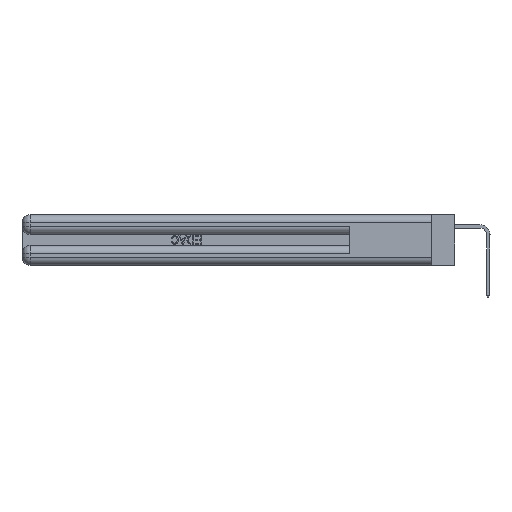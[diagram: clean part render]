
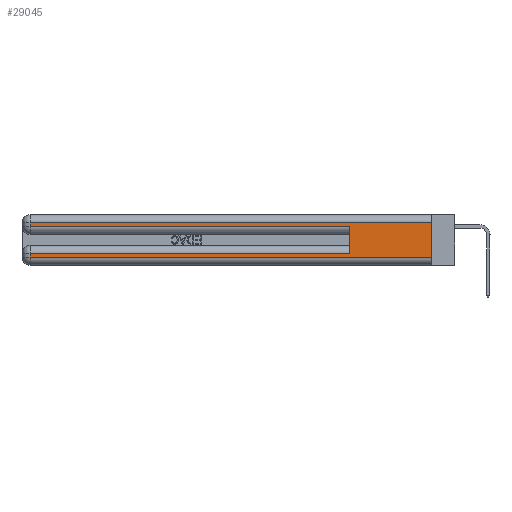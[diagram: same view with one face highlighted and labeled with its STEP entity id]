
A CAD part, left-side view. The second image highlights one B-rep face of the part: STEP entity #29045.
In plain terms, the highlighted planar face has unit normal (-1, 0, 0).
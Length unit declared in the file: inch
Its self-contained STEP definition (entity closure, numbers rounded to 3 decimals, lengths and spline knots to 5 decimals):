
#1526 = ORIENTED_EDGE ( 'NONE', *, *, #7261, .T. ) ;
#1816 = VECTOR ( 'NONE', #19132, 39.37008 ) ;
#1903 = CARTESIAN_POINT ( 'NONE',  ( 0., 0., 0.37 ) ) ;
#2452 = AXIS2_PLACEMENT_3D ( 'NONE', #1903, #26279, #5485 ) ;
#2534 = LINE ( 'NONE', #17965, #29195 ) ;
#3054 = CARTESIAN_POINT ( 'NONE',  ( 0., 0., 0.285 ) ) ;
#3114 = CARTESIAN_POINT ( 'NONE',  ( 0., 2.94, 0.31 ) ) ;
#4350 = ORIENTED_EDGE ( 'NONE', *, *, #4807, .T. ) ;
#4807 = EDGE_CURVE ( 'NONE', #5968, #43733, #16655, .T. ) ;
#5485 = DIRECTION ( 'NONE',  ( 0., 0., -1. ) ) ;
#5968 = VERTEX_POINT ( 'NONE', #27618 ) ;
#6203 = VECTOR ( 'NONE', #27999, 39.37008 ) ;
#6628 = VERTEX_POINT ( 'NONE', #16978 ) ;
#7261 = EDGE_CURVE ( 'NONE', #43733, #33005, #9951, .T. ) ;
#7326 = LINE ( 'NONE', #21052, #6203 ) ;
#8988 = ORIENTED_EDGE ( 'NONE', *, *, #22505, .T. ) ;
#9951 = LINE ( 'NONE', #16258, #11030 ) ;
#10003 = CARTESIAN_POINT ( 'NONE',  ( 0., 0., 0.085 ) ) ;
#10111 = CARTESIAN_POINT ( 'NONE',  ( 0., 2.94, 0.06 ) ) ;
#11030 = VECTOR ( 'NONE', #37002, 39.37008 ) ;
#12995 = EDGE_CURVE ( 'NONE', #5968, #6628, #2534, .T. ) ;
#13821 = CARTESIAN_POINT ( 'NONE',  ( 0., 2.94, 0.285 ) ) ;
#15645 = CARTESIAN_POINT ( 'NONE',  ( 0., 0., 0.06 ) ) ;
#16163 = VERTEX_POINT ( 'NONE', #34158 ) ;
#16258 = CARTESIAN_POINT ( 'NONE',  ( 0., 2.94, 0.37 ) ) ;
#16274 = ORIENTED_EDGE ( 'NONE', *, *, #19928, .T. ) ;
#16655 = LINE ( 'NONE', #18033, #44282 ) ;
#16789 = DIRECTION ( 'NONE',  ( 0., 1., 0. ) ) ;
#16978 = CARTESIAN_POINT ( 'NONE',  ( 0., 0., 0.06 ) ) ;
#17022 = VECTOR ( 'NONE', #27399, 39.37008 ) ;
#17330 = CARTESIAN_POINT ( 'NONE',  ( 0., 0.6, 0.145 ) ) ;
#17733 = VERTEX_POINT ( 'NONE', #29439 ) ;
#17965 = CARTESIAN_POINT ( 'NONE',  ( 0., 0., 0.37 ) ) ;
#18033 = CARTESIAN_POINT ( 'NONE',  ( 0., 0., 0.31 ) ) ;
#18502 = FACE_OUTER_BOUND ( 'NONE', #42942, .T. ) ;
#19132 = DIRECTION ( 'NONE',  ( 0., -1., 0. ) ) ;
#19928 = EDGE_CURVE ( 'NONE', #33005, #17733, #34365, .T. ) ;
#21052 = CARTESIAN_POINT ( 'NONE',  ( 0., 2.94, 0.37 ) ) ;
#21807 = LINE ( 'NONE', #10003, #29906 ) ;
#22505 = EDGE_CURVE ( 'NONE', #27362, #6628, #28496, .T. ) ;
#23562 = ORIENTED_EDGE ( 'NONE', *, *, #42536, .T. ) ;
#24298 = DIRECTION ( 'NONE',  ( 0., 0., 1. ) ) ;
#24777 = DIRECTION ( 'NONE',  ( 0., 0., -1. ) ) ;
#25918 = LINE ( 'NONE', #17330, #43267 ) ;
#26279 = DIRECTION ( 'NONE',  ( 1., 0., 0. ) ) ;
#27362 = VERTEX_POINT ( 'NONE', #10111 ) ;
#27399 = DIRECTION ( 'NONE',  ( 0., -1., 0. ) ) ;
#27618 = CARTESIAN_POINT ( 'NONE',  ( 0., 0., 0.31 ) ) ;
#27999 = DIRECTION ( 'NONE',  ( 0., 0., -1. ) ) ;
#28496 = LINE ( 'NONE', #15645, #1816 ) ;
#28606 = EDGE_CURVE ( 'NONE', #16163, #37944, #21807, .T. ) ;
#29045 = ADVANCED_FACE ( 'NONE', ( #18502 ), #43534, .F. ) ;
#29195 = VECTOR ( 'NONE', #24777, 39.37008 ) ;
#29439 = CARTESIAN_POINT ( 'NONE',  ( 0., 0.6, 0.285 ) ) ;
#29906 = VECTOR ( 'NONE', #16789, 39.37008 ) ;
#30665 = EDGE_CURVE ( 'NONE', #16163, #17733, #25918, .T. ) ;
#33005 = VERTEX_POINT ( 'NONE', #13821 ) ;
#33936 = ORIENTED_EDGE ( 'NONE', *, *, #12995, .F. ) ;
#34158 = CARTESIAN_POINT ( 'NONE',  ( 0., 0.6, 0.085 ) ) ;
#34365 = LINE ( 'NONE', #3054, #17022 ) ;
#35602 = ORIENTED_EDGE ( 'NONE', *, *, #30665, .F. ) ;
#36586 = ORIENTED_EDGE ( 'NONE', *, *, #28606, .T. ) ;
#37002 = DIRECTION ( 'NONE',  ( 0., 0., -1. ) ) ;
#37944 = VERTEX_POINT ( 'NONE', #40193 ) ;
#38784 = DIRECTION ( 'NONE',  ( 0., 1., 0. ) ) ;
#40193 = CARTESIAN_POINT ( 'NONE',  ( 0., 2.94, 0.085 ) ) ;
#42536 = EDGE_CURVE ( 'NONE', #37944, #27362, #7326, .T. ) ;
#42942 = EDGE_LOOP ( 'NONE', ( #33936, #4350, #1526, #16274, #35602, #36586, #23562, #8988 ) ) ;
#43267 = VECTOR ( 'NONE', #24298, 39.37008 ) ;
#43534 = PLANE ( 'NONE',  #2452 ) ;
#43733 = VERTEX_POINT ( 'NONE', #3114 ) ;
#44282 = VECTOR ( 'NONE', #38784, 39.37008 ) ;
